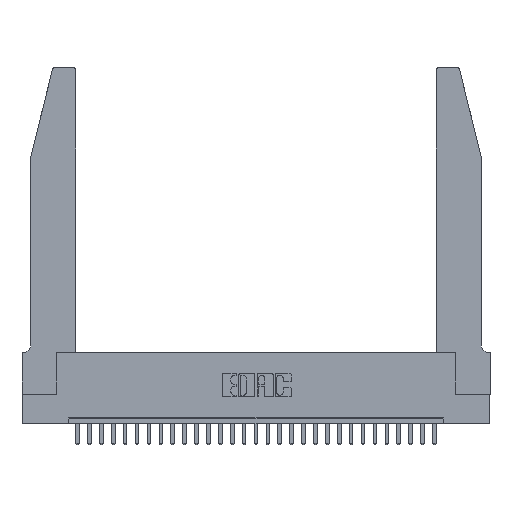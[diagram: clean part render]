
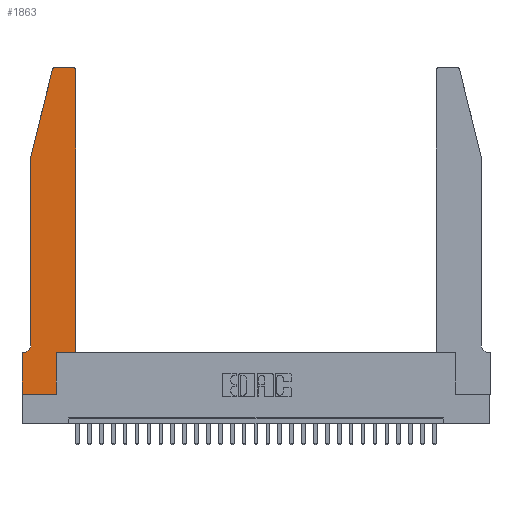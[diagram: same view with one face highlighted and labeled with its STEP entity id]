
A CAD part, top view. The second image highlights one B-rep face of the part: STEP entity #1863.
In plain terms, the highlighted planar face has unit normal (0, 0, 1).
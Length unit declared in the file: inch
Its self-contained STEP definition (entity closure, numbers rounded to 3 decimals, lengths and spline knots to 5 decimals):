
#101 = CARTESIAN_POINT ( 'NONE',  ( 0., 0., 0.37 ) ) ;
#105 = PLANE ( 'NONE',  #1127 ) ;
#224 = CARTESIAN_POINT ( 'NONE',  ( 0.284, 2.75, 0.37 ) ) ;
#227 = DIRECTION ( 'NONE',  ( -1., 0., 0. ) ) ;
#258 = CARTESIAN_POINT ( 'NONE',  ( 0.25487, 2.72718, 0.37 ) ) ;
#379 = DIRECTION ( 'NONE',  ( 0., -1., 0. ) ) ;
#683 = VERTEX_POINT ( 'NONE', #9234 ) ;
#970 = VERTEX_POINT ( 'NONE', #12763 ) ;
#1055 = ORIENTED_EDGE ( 'NONE', *, *, #2383, .T. ) ;
#1127 = AXIS2_PLACEMENT_3D ( 'NONE', #2427, #6638, #18459 ) ;
#1157 = CARTESIAN_POINT ( 'NONE',  ( 0.0755, 0.35, 0.37 ) ) ;
#1863 = ADVANCED_FACE ( 'NONE', ( #3722 ), #105, .T. ) ;
#1943 = VECTOR ( 'NONE', #379, 39.37008 ) ;
#2316 = CIRCLE ( 'NONE', #19695, 0.03 ) ;
#2383 = EDGE_CURVE ( 'NONE', #18362, #15835, #12738, .T. ) ;
#2427 = CARTESIAN_POINT ( 'NONE',  ( 0., 0.35, 0.37 ) ) ;
#2643 = DIRECTION ( 'NONE',  ( 0., 0., -1. ) ) ;
#2901 = ORIENTED_EDGE ( 'NONE', *, *, #22881, .T. ) ;
#3184 = ORIENTED_EDGE ( 'NONE', *, *, #29185, .T. ) ;
#3204 = ORIENTED_EDGE ( 'NONE', *, *, #25908, .T. ) ;
#3329 = ORIENTED_EDGE ( 'NONE', *, *, #6897, .T. ) ;
#3722 = FACE_OUTER_BOUND ( 'NONE', #9087, .T. ) ;
#4130 = CARTESIAN_POINT ( 'NONE',  ( 0.0755, 2., 0.37 ) ) ;
#4291 = CARTESIAN_POINT ( 'NONE',  ( 0.2865, 0., 0.37 ) ) ;
#4331 = CARTESIAN_POINT ( 'NONE',  ( 0.4505, 2.72, 0.37 ) ) ;
#4603 = EDGE_CURVE ( 'NONE', #21707, #18362, #11109, .T. ) ;
#5548 = VERTEX_POINT ( 'NONE', #224 ) ;
#5580 = DIRECTION ( 'NONE',  ( 0., 1., 0. ) ) ;
#5835 = CARTESIAN_POINT ( 'NONE',  ( 0.0755, 0.42, 0.37 ) ) ;
#5970 = CARTESIAN_POINT ( 'NONE',  ( 0.4505, 0.35, 0.37 ) ) ;
#6248 = DIRECTION ( 'NONE',  ( 1., 0., 0. ) ) ;
#6638 = DIRECTION ( 'NONE',  ( 0., 0., 1. ) ) ;
#6897 = EDGE_CURVE ( 'NONE', #15835, #18841, #29246, .T. ) ;
#7610 = VECTOR ( 'NONE', #5580, 39.37008 ) ;
#7724 = ORIENTED_EDGE ( 'NONE', *, *, #20217, .T. ) ;
#7726 = VERTEX_POINT ( 'NONE', #4291 ) ;
#7952 = LINE ( 'NONE', #28107, #13342 ) ;
#7993 = EDGE_CURVE ( 'NONE', #5548, #21707, #2316, .T. ) ;
#8002 = ORIENTED_EDGE ( 'NONE', *, *, #7993, .T. ) ;
#8192 = VERTEX_POINT ( 'NONE', #13675 ) ;
#8398 = CARTESIAN_POINT ( 'NONE',  ( 0.0755, 2., 0.37 ) ) ;
#8598 = CARTESIAN_POINT ( 'NONE',  ( 0.2865, 0.35, 0.37 ) ) ;
#8669 = LINE ( 'NONE', #5970, #7610 ) ;
#8758 = DIRECTION ( 'NONE',  ( 1., 0., 0. ) ) ;
#8799 = LINE ( 'NONE', #101, #12059 ) ;
#9087 = EDGE_LOOP ( 'NONE', ( #7724, #8002, #23533, #1055, #3329, #3204, #2901, #18372, #9756, #20406, #14919, #3184 ) ) ;
#9234 = CARTESIAN_POINT ( 'NONE',  ( 0.4205, 2.75, 0.37 ) ) ;
#9756 = ORIENTED_EDGE ( 'NONE', *, *, #25922, .T. ) ;
#9867 = AXIS2_PLACEMENT_3D ( 'NONE', #17604, #13100, #6248 ) ;
#11104 = VECTOR ( 'NONE', #8758, 39.37008 ) ;
#11109 = LINE ( 'NONE', #8398, #27231 ) ;
#11604 = DIRECTION ( 'NONE',  ( 1., 0., 0. ) ) ;
#11749 = EDGE_CURVE ( 'NONE', #17076, #8192, #17205, .T. ) ;
#11807 = CARTESIAN_POINT ( 'NONE',  ( 0.0055, 0.42, 0.37 ) ) ;
#12059 = VECTOR ( 'NONE', #22777, 39.37008 ) ;
#12657 = DIRECTION ( 'NONE',  ( -1., 0., 0. ) ) ;
#12738 = LINE ( 'NONE', #23200, #1943 ) ;
#12763 = CARTESIAN_POINT ( 'NONE',  ( 0., 0.35, 0.37 ) ) ;
#13100 = DIRECTION ( 'NONE',  ( 0., 0., 1. ) ) ;
#13324 = AXIS2_PLACEMENT_3D ( 'NONE', #11807, #2643, #227 ) ;
#13342 = VECTOR ( 'NONE', #14425, 39.37008 ) ;
#13675 = CARTESIAN_POINT ( 'NONE',  ( 0.4505, 0.35, 0.37 ) ) ;
#14425 = DIRECTION ( 'NONE',  ( 1., 0., 0. ) ) ;
#14919 = ORIENTED_EDGE ( 'NONE', *, *, #25429, .T. ) ;
#15835 = VERTEX_POINT ( 'NONE', #5835 ) ;
#16103 = DIRECTION ( 'NONE',  ( 0., 0., 1. ) ) ;
#16543 = VECTOR ( 'NONE', #17391, 39.37008 ) ;
#17076 = VERTEX_POINT ( 'NONE', #8598 ) ;
#17205 = LINE ( 'NONE', #22032, #11104 ) ;
#17252 = CIRCLE ( 'NONE', #9867, 0.03 ) ;
#17391 = DIRECTION ( 'NONE',  ( -1., 0., 0. ) ) ;
#17604 = CARTESIAN_POINT ( 'NONE',  ( 0.4205, 2.72, 0.37 ) ) ;
#17817 = DIRECTION ( 'NONE',  ( -0.239, -0.971, 0. ) ) ;
#18362 = VERTEX_POINT ( 'NONE', #4130 ) ;
#18372 = ORIENTED_EDGE ( 'NONE', *, *, #28801, .T. ) ;
#18459 = DIRECTION ( 'NONE',  ( 1., 0., 0. ) ) ;
#18841 = VERTEX_POINT ( 'NONE', #28587 ) ;
#19535 = VERTEX_POINT ( 'NONE', #23259 ) ;
#19695 = AXIS2_PLACEMENT_3D ( 'NONE', #25300, #16103, #11604 ) ;
#19696 = DIRECTION ( 'NONE',  ( 0., 1., 0. ) ) ;
#20217 = EDGE_CURVE ( 'NONE', #683, #5548, #26640, .T. ) ;
#20406 = ORIENTED_EDGE ( 'NONE', *, *, #11749, .T. ) ;
#20605 = VECTOR ( 'NONE', #12657, 39.37008 ) ;
#21676 = CARTESIAN_POINT ( 'NONE',  ( 0.2605, 2.75, 0.37 ) ) ;
#21707 = VERTEX_POINT ( 'NONE', #258 ) ;
#21960 = VECTOR ( 'NONE', #19696, 39.37008 ) ;
#22032 = CARTESIAN_POINT ( 'NONE',  ( 0.4505, 0.35, 0.37 ) ) ;
#22126 = VERTEX_POINT ( 'NONE', #4331 ) ;
#22777 = DIRECTION ( 'NONE',  ( 0., -1., 0. ) ) ;
#22881 = EDGE_CURVE ( 'NONE', #970, #19535, #8799, .T. ) ;
#22990 = LINE ( 'NONE', #26478, #21960 ) ;
#23200 = CARTESIAN_POINT ( 'NONE',  ( 0.0755, 2., 0.37 ) ) ;
#23259 = CARTESIAN_POINT ( 'NONE',  ( 0., 0., 0.37 ) ) ;
#23533 = ORIENTED_EDGE ( 'NONE', *, *, #4603, .T. ) ;
#25300 = CARTESIAN_POINT ( 'NONE',  ( 0.284, 2.72, 0.37 ) ) ;
#25429 = EDGE_CURVE ( 'NONE', #8192, #22126, #8669, .T. ) ;
#25838 = LINE ( 'NONE', #1157, #16543 ) ;
#25908 = EDGE_CURVE ( 'NONE', #18841, #970, #25838, .T. ) ;
#25922 = EDGE_CURVE ( 'NONE', #7726, #17076, #22990, .T. ) ;
#26478 = CARTESIAN_POINT ( 'NONE',  ( 0.2865, 0.35, 0.37 ) ) ;
#26640 = LINE ( 'NONE', #21676, #20605 ) ;
#27231 = VECTOR ( 'NONE', #17817, 39.37008 ) ;
#28107 = CARTESIAN_POINT ( 'NONE',  ( 0., 0., 0.37 ) ) ;
#28587 = CARTESIAN_POINT ( 'NONE',  ( 0.0055, 0.35, 0.37 ) ) ;
#28801 = EDGE_CURVE ( 'NONE', #19535, #7726, #7952, .T. ) ;
#29185 = EDGE_CURVE ( 'NONE', #22126, #683, #17252, .T. ) ;
#29246 = CIRCLE ( 'NONE', #13324, 0.07 ) ;
